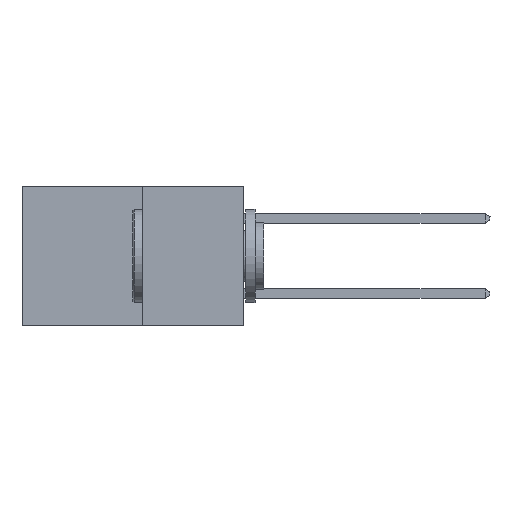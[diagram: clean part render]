
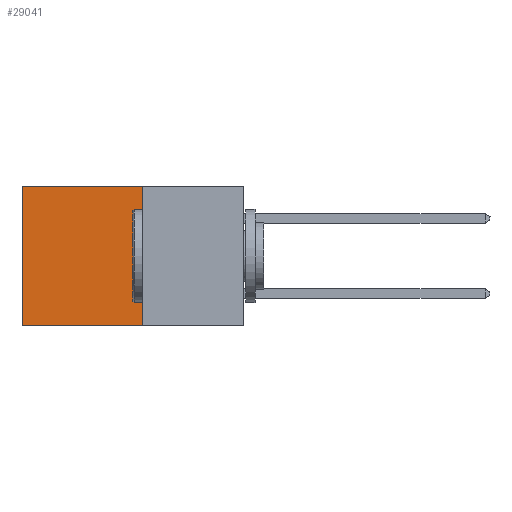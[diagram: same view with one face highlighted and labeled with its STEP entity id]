
A CAD part, left-side view. The second image highlights one B-rep face of the part: STEP entity #29041.
In plain terms, the highlighted planar face has unit normal (-1, 0, 0).
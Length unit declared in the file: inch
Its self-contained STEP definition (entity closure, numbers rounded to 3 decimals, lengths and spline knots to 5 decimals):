
#143 = LINE ( 'NONE', #9365, #4088 ) ;
#2103 = ORIENTED_EDGE ( 'NONE', *, *, #27192, .F. ) ;
#2267 = DIRECTION ( 'NONE',  ( 0., 0., -1. ) ) ;
#2614 = VERTEX_POINT ( 'NONE', #28530 ) ;
#2780 = ORIENTED_EDGE ( 'NONE', *, *, #28929, .T. ) ;
#4088 = VECTOR ( 'NONE', #27677, 39.37008 ) ;
#4610 = CARTESIAN_POINT ( 'NONE',  ( 0.277, 0.27, 0. ) ) ;
#5186 = EDGE_LOOP ( 'NONE', ( #2780, #7822, #2103, #15160 ) ) ;
#6695 = CARTESIAN_POINT ( 'NONE',  ( 0.277, 0.27, -0.37 ) ) ;
#7822 = ORIENTED_EDGE ( 'NONE', *, *, #18470, .F. ) ;
#8083 = VECTOR ( 'NONE', #13446, 39.37008 ) ;
#8997 = VECTOR ( 'NONE', #22921, 39.37008 ) ;
#9365 = CARTESIAN_POINT ( 'NONE',  ( 0.277, 0.27, -0.37 ) ) ;
#9727 = LINE ( 'NONE', #4610, #8997 ) ;
#10392 = CARTESIAN_POINT ( 'NONE',  ( 0.277, 0.59, -0.37 ) ) ;
#11145 = CARTESIAN_POINT ( 'NONE',  ( 0.277, 0.59, -0.37 ) ) ;
#11839 = DIRECTION ( 'NONE',  ( 0., 0., -1. ) ) ;
#13410 = VERTEX_POINT ( 'NONE', #10392 ) ;
#13415 = CARTESIAN_POINT ( 'NONE',  ( 0.277, 0.27, 0. ) ) ;
#13446 = DIRECTION ( 'NONE',  ( 0., 0., -1. ) ) ;
#14202 = LINE ( 'NONE', #11145, #8083 ) ;
#15160 = ORIENTED_EDGE ( 'NONE', *, *, #21268, .T. ) ;
#15987 = DIRECTION ( 'NONE',  ( 1., 0., 0. ) ) ;
#18190 = VERTEX_POINT ( 'NONE', #22050 ) ;
#18470 = EDGE_CURVE ( 'NONE', #18190, #13410, #143, .T. ) ;
#18903 = LINE ( 'NONE', #27793, #19611 ) ;
#18932 = PLANE ( 'NONE',  #21171 ) ;
#19611 = VECTOR ( 'NONE', #11839, 39.37008 ) ;
#21171 = AXIS2_PLACEMENT_3D ( 'NONE', #6695, #15987, #2267 ) ;
#21268 = EDGE_CURVE ( 'NONE', #21615, #2614, #9727, .T. ) ;
#21615 = VERTEX_POINT ( 'NONE', #13415 ) ;
#22050 = CARTESIAN_POINT ( 'NONE',  ( 0.277, 0.27, -0.37 ) ) ;
#22921 = DIRECTION ( 'NONE',  ( 0., 1., 0. ) ) ;
#23433 = FACE_OUTER_BOUND ( 'NONE', #5186, .T. ) ;
#27192 = EDGE_CURVE ( 'NONE', #21615, #18190, #18903, .T. ) ;
#27677 = DIRECTION ( 'NONE',  ( 0., 1., 0. ) ) ;
#27793 = CARTESIAN_POINT ( 'NONE',  ( 0.277, 0.27, -0.37 ) ) ;
#28530 = CARTESIAN_POINT ( 'NONE',  ( 0.277, 0.59, 0. ) ) ;
#28929 = EDGE_CURVE ( 'NONE', #2614, #13410, #14202, .T. ) ;
#29041 = ADVANCED_FACE ( 'NONE', ( #23433 ), #18932, .F. ) ;
